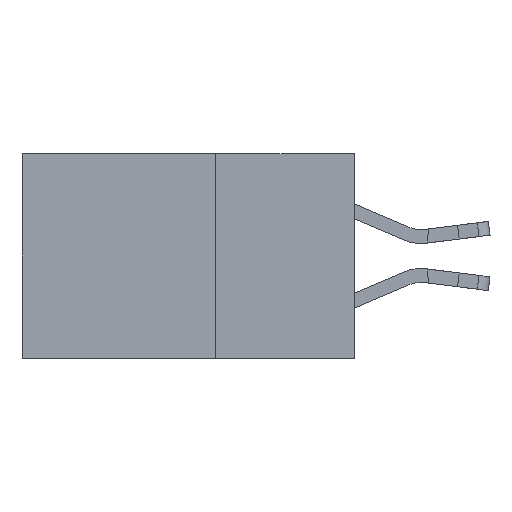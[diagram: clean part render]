
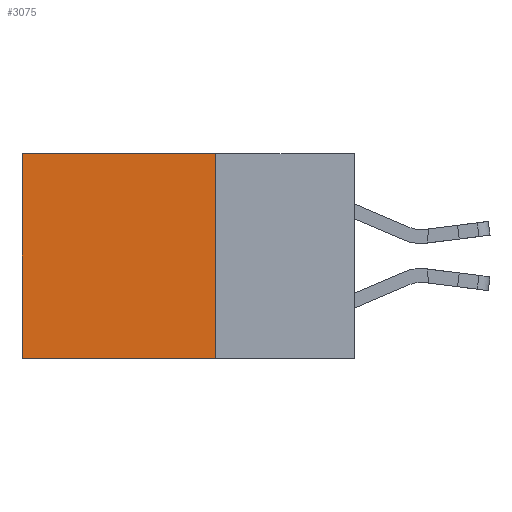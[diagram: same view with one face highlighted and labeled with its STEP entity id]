
A CAD part, left-side view. The second image highlights one B-rep face of the part: STEP entity #3075.
In plain terms, the highlighted planar face has unit normal (-1, 0, 0).
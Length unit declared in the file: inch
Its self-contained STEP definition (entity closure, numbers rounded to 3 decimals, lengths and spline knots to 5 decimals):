
#893 = CARTESIAN_POINT ( 'NONE',  ( 0.298, 0.25, 0. ) ) ;
#1143 = CARTESIAN_POINT ( 'NONE',  ( 0.298, 0.6, 0. ) ) ;
#1389 = CARTESIAN_POINT ( 'NONE',  ( 0.298, 0.6, 0. ) ) ;
#1635 = VERTEX_POINT ( 'NONE', #12231 ) ;
#3075 = ADVANCED_FACE ( 'NONE', ( #6096 ), #6690, .F. ) ;
#3414 = AXIS2_PLACEMENT_3D ( 'NONE', #10257, #6212, #9360 ) ;
#4154 = EDGE_CURVE ( 'NONE', #11690, #12326, #19160, .T. ) ;
#5106 = LINE ( 'NONE', #1389, #17557 ) ;
#6096 = FACE_OUTER_BOUND ( 'NONE', #10449, .T. ) ;
#6212 = DIRECTION ( 'NONE',  ( 1., 0., 0. ) ) ;
#6649 = ORIENTED_EDGE ( 'NONE', *, *, #14043, .T. ) ;
#6690 = PLANE ( 'NONE',  #3414 ) ;
#7443 = CARTESIAN_POINT ( 'NONE',  ( 0.298, 0.25, 0. ) ) ;
#7649 = DIRECTION ( 'NONE',  ( 0., 1., 0. ) ) ;
#9360 = DIRECTION ( 'NONE',  ( 0., 0., -1. ) ) ;
#9477 = VECTOR ( 'NONE', #7649, 39.37008 ) ;
#9759 = EDGE_CURVE ( 'NONE', #12326, #1635, #16450, .T. ) ;
#10257 = CARTESIAN_POINT ( 'NONE',  ( 0.298, 0.25, 0. ) ) ;
#10449 = EDGE_LOOP ( 'NONE', ( #10906, #10930, #15103, #6649 ) ) ;
#10669 = VECTOR ( 'NONE', #18684, 39.37008 ) ;
#10906 = ORIENTED_EDGE ( 'NONE', *, *, #18941, .T. ) ;
#10930 = ORIENTED_EDGE ( 'NONE', *, *, #9759, .F. ) ;
#11068 = DIRECTION ( 'NONE',  ( 0., 1., 0. ) ) ;
#11690 = VERTEX_POINT ( 'NONE', #15263 ) ;
#11720 = VECTOR ( 'NONE', #11068, 39.37008 ) ;
#12231 = CARTESIAN_POINT ( 'NONE',  ( 0.298, 0.6, -0.37 ) ) ;
#12326 = VERTEX_POINT ( 'NONE', #19603 ) ;
#13134 = DIRECTION ( 'NONE',  ( 0., 0., -1. ) ) ;
#13828 = LINE ( 'NONE', #893, #9477 ) ;
#14043 = EDGE_CURVE ( 'NONE', #11690, #17256, #13828, .T. ) ;
#15103 = ORIENTED_EDGE ( 'NONE', *, *, #4154, .F. ) ;
#15263 = CARTESIAN_POINT ( 'NONE',  ( 0.298, 0.25, 0. ) ) ;
#16450 = LINE ( 'NONE', #19012, #11720 ) ;
#17256 = VERTEX_POINT ( 'NONE', #1143 ) ;
#17557 = VECTOR ( 'NONE', #13134, 39.37008 ) ;
#18684 = DIRECTION ( 'NONE',  ( 0., 0., -1. ) ) ;
#18941 = EDGE_CURVE ( 'NONE', #17256, #1635, #5106, .T. ) ;
#19012 = CARTESIAN_POINT ( 'NONE',  ( 0.298, 0.25, -0.37 ) ) ;
#19160 = LINE ( 'NONE', #7443, #10669 ) ;
#19603 = CARTESIAN_POINT ( 'NONE',  ( 0.298, 0.25, -0.37 ) ) ;
